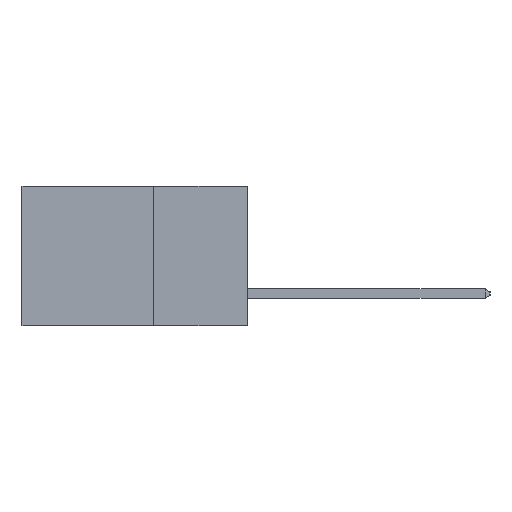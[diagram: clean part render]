
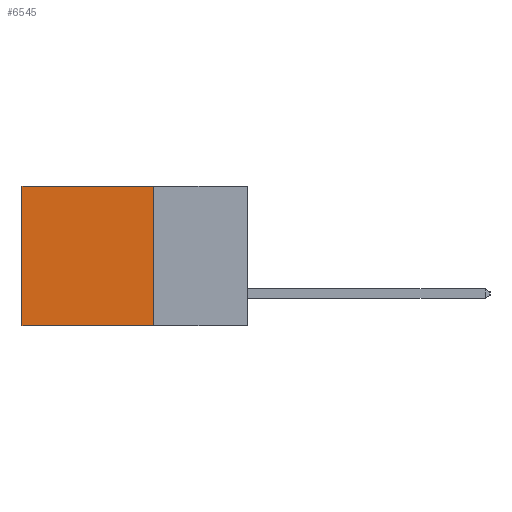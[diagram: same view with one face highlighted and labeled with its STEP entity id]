
A CAD part, left-side view. The second image highlights one B-rep face of the part: STEP entity #6545.
In plain terms, the highlighted planar face has unit normal (-1, 0, 0).
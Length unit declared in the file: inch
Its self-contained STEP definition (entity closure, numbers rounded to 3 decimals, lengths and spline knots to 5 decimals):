
#84 = VERTEX_POINT ( 'NONE', #4088 ) ;
#1188 = DIRECTION ( 'NONE',  ( 0., 1., 0. ) ) ;
#1248 = CARTESIAN_POINT ( 'NONE',  ( 0.2615, 0.25, 0. ) ) ;
#1314 = DIRECTION ( 'NONE',  ( 0., 1., 0. ) ) ;
#2834 = CARTESIAN_POINT ( 'NONE',  ( 0.2615, 0.25, -0.37 ) ) ;
#3493 = DIRECTION ( 'NONE',  ( 0., 0., -1. ) ) ;
#3496 = CARTESIAN_POINT ( 'NONE',  ( 0.2615, 0.25, -0.37 ) ) ;
#4088 = CARTESIAN_POINT ( 'NONE',  ( 0.2615, 0.6, -0.37 ) ) ;
#4091 = VERTEX_POINT ( 'NONE', #11022 ) ;
#4369 = CARTESIAN_POINT ( 'NONE',  ( 0.2615, 0.6, 0. ) ) ;
#4642 = AXIS2_PLACEMENT_3D ( 'NONE', #19783, #8122, #5315 ) ;
#5068 = VECTOR ( 'NONE', #1188, 39.37008 ) ;
#5315 = DIRECTION ( 'NONE',  ( 0., 0., -1. ) ) ;
#5354 = EDGE_CURVE ( 'NONE', #4091, #18735, #11976, .T. ) ;
#5517 = ORIENTED_EDGE ( 'NONE', *, *, #15775, .T. ) ;
#6389 = VERTEX_POINT ( 'NONE', #4369 ) ;
#6545 = ADVANCED_FACE ( 'NONE', ( #7360 ), #19719, .F. ) ;
#6659 = LINE ( 'NONE', #1248, #14756 ) ;
#7360 = FACE_OUTER_BOUND ( 'NONE', #13190, .T. ) ;
#7890 = ORIENTED_EDGE ( 'NONE', *, *, #15218, .T. ) ;
#8122 = DIRECTION ( 'NONE',  ( 1., 0., 0. ) ) ;
#8184 = VECTOR ( 'NONE', #3493, 39.37008 ) ;
#11022 = CARTESIAN_POINT ( 'NONE',  ( 0.2615, 0.25, 0. ) ) ;
#11712 = LINE ( 'NONE', #15892, #15944 ) ;
#11976 = LINE ( 'NONE', #3496, #8184 ) ;
#12764 = EDGE_CURVE ( 'NONE', #18735, #84, #14741, .T. ) ;
#13190 = EDGE_LOOP ( 'NONE', ( #5517, #18089, #19895, #7890 ) ) ;
#14741 = LINE ( 'NONE', #2834, #5068 ) ;
#14756 = VECTOR ( 'NONE', #1314, 39.37008 ) ;
#15218 = EDGE_CURVE ( 'NONE', #4091, #6389, #6659, .T. ) ;
#15646 = DIRECTION ( 'NONE',  ( 0., 0., -1. ) ) ;
#15775 = EDGE_CURVE ( 'NONE', #6389, #84, #11712, .T. ) ;
#15892 = CARTESIAN_POINT ( 'NONE',  ( 0.2615, 0.6, -0.37 ) ) ;
#15944 = VECTOR ( 'NONE', #15646, 39.37008 ) ;
#16875 = CARTESIAN_POINT ( 'NONE',  ( 0.2615, 0.25, -0.37 ) ) ;
#18089 = ORIENTED_EDGE ( 'NONE', *, *, #12764, .F. ) ;
#18735 = VERTEX_POINT ( 'NONE', #16875 ) ;
#19719 = PLANE ( 'NONE',  #4642 ) ;
#19783 = CARTESIAN_POINT ( 'NONE',  ( 0.2615, 0.25, -0.37 ) ) ;
#19895 = ORIENTED_EDGE ( 'NONE', *, *, #5354, .F. ) ;
